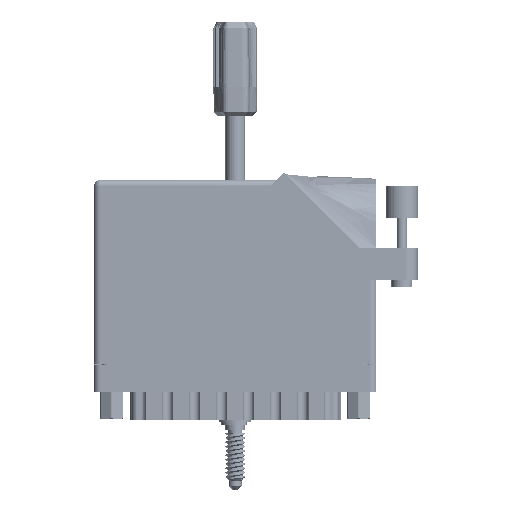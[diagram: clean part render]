
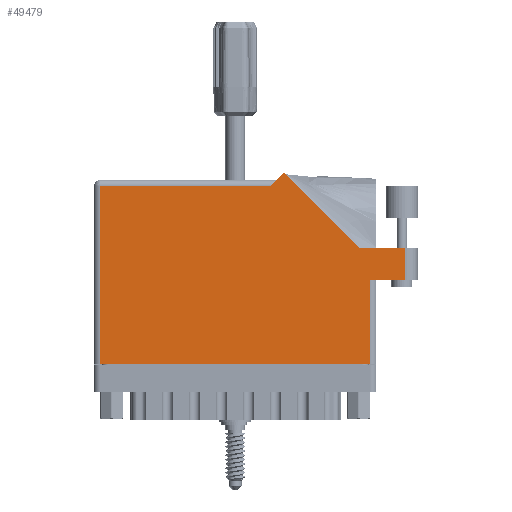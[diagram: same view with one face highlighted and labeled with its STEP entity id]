
A CAD part, front view. The second image highlights one B-rep face of the part: STEP entity #49479.
In plain terms, the highlighted face is planar.
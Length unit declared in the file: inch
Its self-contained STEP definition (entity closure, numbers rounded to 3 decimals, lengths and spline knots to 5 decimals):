
#168 = VERTEX_POINT ( 'NONE', #55754 ) ;
#1148 = LINE ( 'NONE', #57440, #16694 ) ;
#1992 = LINE ( 'NONE', #63804, #29514 ) ;
#3324 = CARTESIAN_POINT ( 'NONE',  ( 1.82871, 1.84571, 0. ) ) ;
#3825 = CARTESIAN_POINT ( 'NONE',  ( 0., 1.775, 0. ) ) ;
#5318 = ORIENTED_EDGE ( 'NONE', *, *, #25620, .T. ) ;
#7267 = ORIENTED_EDGE ( 'NONE', *, *, #35438, .T. ) ;
#9261 = LINE ( 'NONE', #11657, #60744 ) ;
#9533 = EDGE_CURVE ( 'NONE', #66503, #84063, #9261, .T. ) ;
#10112 = CARTESIAN_POINT ( 'NONE',  ( 2.656, 0.815, 0. ) ) ;
#10780 = VERTEX_POINT ( 'NONE', #10112 ) ;
#11088 = CARTESIAN_POINT ( 'NONE',  ( 0.062, 1.713, 0. ) ) ;
#11657 = CARTESIAN_POINT ( 'NONE',  ( 0., 1.713, 0. ) ) ;
#13407 = CARTESIAN_POINT ( 'NONE',  ( 0., 0., 0. ) ) ;
#14897 = LINE ( 'NONE', #31336, #93958 ) ;
#15825 = EDGE_CURVE ( 'NONE', #10780, #59602, #82518, .T. ) ;
#15949 = EDGE_CURVE ( 'NONE', #88745, #98401, #90952, .T. ) ;
#16694 = VECTOR ( 'NONE', #26587, 39.37008 ) ;
#20584 = EDGE_LOOP ( 'NONE', ( #22836, #7267, #70127, #22655, #23791, #54241, #5318, #27727, #50841 ) ) ;
#21520 = EDGE_CURVE ( 'NONE', #98401, #66503, #1148, .T. ) ;
#21947 = AXIS2_PLACEMENT_3D ( 'NONE', #3825, #80118, #34236 ) ;
#22655 = ORIENTED_EDGE ( 'NONE', *, *, #15949, .T. ) ;
#22836 = ORIENTED_EDGE ( 'NONE', *, *, #15825, .T. ) ;
#23791 = ORIENTED_EDGE ( 'NONE', *, *, #21520, .T. ) ;
#25620 = EDGE_CURVE ( 'NONE', #84063, #168, #64724, .T. ) ;
#26587 = DIRECTION ( 'NONE',  ( -0.707, -0.707, 0. ) ) ;
#27727 = ORIENTED_EDGE ( 'NONE', *, *, #46358, .T. ) ;
#29514 = VECTOR ( 'NONE', #47687, 39.37008 ) ;
#31336 = CARTESIAN_POINT ( 'NONE',  ( 2.656, 0.815, 0. ) ) ;
#34236 = DIRECTION ( 'NONE',  ( -1., 0., 0. ) ) ;
#35438 = EDGE_CURVE ( 'NONE', #59602, #89603, #70011, .T. ) ;
#39471 = CARTESIAN_POINT ( 'NONE',  ( 2.55242, 1.122, 0. ) ) ;
#42342 = DIRECTION ( 'NONE',  ( 1., 0., 0. ) ) ;
#46358 = EDGE_CURVE ( 'NONE', #168, #63397, #57347, .T. ) ;
#46562 = CARTESIAN_POINT ( 'NONE',  ( 0.062, 0., 0. ) ) ;
#47236 = CARTESIAN_POINT ( 'NONE',  ( 2.993, 1.122, 0. ) ) ;
#47687 = DIRECTION ( 'NONE',  ( -1., 0., 0. ) ) ;
#49479 = ADVANCED_FACE ( 'NONE', ( #58393 ), #65023, .F. ) ;
#49720 = DIRECTION ( 'NONE',  ( 0., 1., 0. ) ) ;
#50171 = DIRECTION ( 'NONE',  ( -1., 0., 0. ) ) ;
#50819 = EDGE_CURVE ( 'NONE', #89603, #88745, #1992, .T. ) ;
#50841 = ORIENTED_EDGE ( 'NONE', *, *, #65331, .T. ) ;
#53980 = CARTESIAN_POINT ( 'NONE',  ( 1.696, 1.713, 0. ) ) ;
#54241 = ORIENTED_EDGE ( 'NONE', *, *, #9533, .T. ) ;
#55094 = CARTESIAN_POINT ( 'NONE',  ( 2.993, 0.815, 0. ) ) ;
#55754 = CARTESIAN_POINT ( 'NONE',  ( 0.062, 0., 0. ) ) ;
#57347 = LINE ( 'NONE', #13407, #76453 ) ;
#57440 = CARTESIAN_POINT ( 'NONE',  ( 1.758, 1.775, 0. ) ) ;
#58393 = FACE_OUTER_BOUND ( 'NONE', #20584, .T. ) ;
#59602 = VERTEX_POINT ( 'NONE', #55094 ) ;
#60744 = VECTOR ( 'NONE', #50171, 39.37008 ) ;
#62654 = CARTESIAN_POINT ( 'NONE',  ( 2.718, 0.815, 0. ) ) ;
#63397 = VERTEX_POINT ( 'NONE', #73404 ) ;
#63804 = CARTESIAN_POINT ( 'NONE',  ( 3.118, 1.122, 0. ) ) ;
#64724 = LINE ( 'NONE', #46562, #80326 ) ;
#65023 = PLANE ( 'NONE',  #21947 ) ;
#65331 = EDGE_CURVE ( 'NONE', #63397, #10780, #14897, .T. ) ;
#66503 = VERTEX_POINT ( 'NONE', #53980 ) ;
#70011 = LINE ( 'NONE', #87850, #73570 ) ;
#70127 = ORIENTED_EDGE ( 'NONE', *, *, #50819, .T. ) ;
#73404 = CARTESIAN_POINT ( 'NONE',  ( 2.656, 0., 0. ) ) ;
#73570 = VECTOR ( 'NONE', #49720, 39.37008 ) ;
#76453 = VECTOR ( 'NONE', #42342, 39.37008 ) ;
#76603 = DIRECTION ( 'NONE',  ( 0., 1., 0. ) ) ;
#77390 = DIRECTION ( 'NONE',  ( 1., 0., 0. ) ) ;
#78148 = DIRECTION ( 'NONE',  ( -0.707, 0.707, 0. ) ) ;
#80118 = DIRECTION ( 'NONE',  ( 0., 0., -1. ) ) ;
#80326 = VECTOR ( 'NONE', #85378, 39.37008 ) ;
#82518 = LINE ( 'NONE', #62654, #93337 ) ;
#84063 = VERTEX_POINT ( 'NONE', #11088 ) ;
#85378 = DIRECTION ( 'NONE',  ( 0., -1., 0. ) ) ;
#85497 = CARTESIAN_POINT ( 'NONE',  ( 2.55242, 1.122, 0. ) ) ;
#87850 = CARTESIAN_POINT ( 'NONE',  ( 2.993, 1.122, 0. ) ) ;
#88745 = VERTEX_POINT ( 'NONE', #39471 ) ;
#89603 = VERTEX_POINT ( 'NONE', #47236 ) ;
#90952 = LINE ( 'NONE', #85497, #95694 ) ;
#93337 = VECTOR ( 'NONE', #77390, 39.37008 ) ;
#93958 = VECTOR ( 'NONE', #76603, 39.37008 ) ;
#95694 = VECTOR ( 'NONE', #78148, 39.37008 ) ;
#98401 = VERTEX_POINT ( 'NONE', #3324 ) ;
